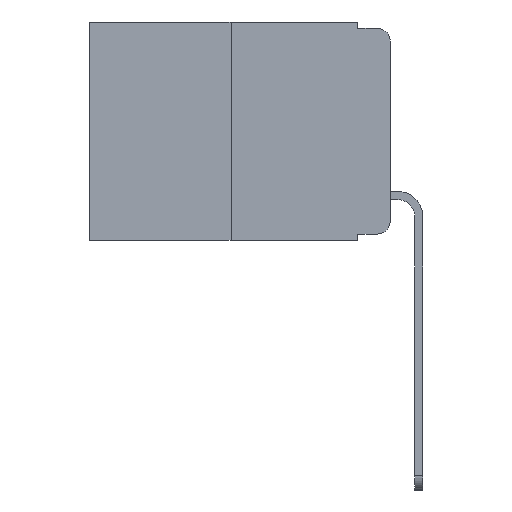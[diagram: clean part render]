
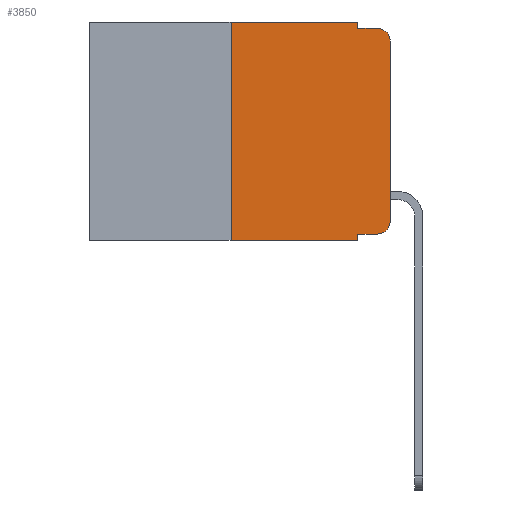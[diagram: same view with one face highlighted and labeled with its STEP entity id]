
A CAD part, left-side view. The second image highlights one B-rep face of the part: STEP entity #3850.
In plain terms, the highlighted planar face has unit normal (-1, 0, 0).
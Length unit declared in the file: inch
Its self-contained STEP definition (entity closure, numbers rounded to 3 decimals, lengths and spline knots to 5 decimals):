
#22 = VERTEX_POINT ( 'NONE', #5434 ) ;
#268 = LINE ( 'NONE', #22617, #21982 ) ;
#506 = CARTESIAN_POINT ( 'NONE',  ( 0., 0.051, -0.01 ) ) ;
#622 = EDGE_CURVE ( 'NONE', #5404, #12335, #5553, .T. ) ;
#743 = CARTESIAN_POINT ( 'NONE',  ( 0., 0.02, -0.333 ) ) ;
#933 = VERTEX_POINT ( 'NONE', #16867 ) ;
#1310 = LINE ( 'NONE', #3900, #15167 ) ;
#1451 = CARTESIAN_POINT ( 'NONE',  ( 0., 0.02, -0.313 ) ) ;
#2582 = CARTESIAN_POINT ( 'NONE',  ( 0., 0.051, -0.333 ) ) ;
#2832 = EDGE_CURVE ( 'NONE', #20714, #9793, #21020, .T. ) ;
#3211 = DIRECTION ( 'NONE',  ( 0., 0., -1. ) ) ;
#3547 = VERTEX_POINT ( 'NONE', #15795 ) ;
#3850 = ADVANCED_FACE ( 'NONE', ( #6837 ), #14515, .F. ) ;
#3899 = LINE ( 'NONE', #9962, #21106 ) ;
#3900 = CARTESIAN_POINT ( 'NONE',  ( 0., 0., 0. ) ) ;
#3973 = CARTESIAN_POINT ( 'NONE',  ( 0., 0., -0.313 ) ) ;
#4809 = CARTESIAN_POINT ( 'NONE',  ( 0., 0.02, -0.03 ) ) ;
#4933 = VECTOR ( 'NONE', #21950, 39.37008 ) ;
#5178 = DIRECTION ( 'NONE',  ( 0., -1., 0. ) ) ;
#5259 = LINE ( 'NONE', #506, #13717 ) ;
#5337 = VERTEX_POINT ( 'NONE', #8022 ) ;
#5404 = VERTEX_POINT ( 'NONE', #743 ) ;
#5434 = CARTESIAN_POINT ( 'NONE',  ( 0., 0.02, -0.01 ) ) ;
#5553 = CIRCLE ( 'NONE', #9701, 0.02 ) ;
#5694 = LINE ( 'NONE', #6574, #15062 ) ;
#6097 = CARTESIAN_POINT ( 'NONE',  ( 0., 0.051, -0.343 ) ) ;
#6574 = CARTESIAN_POINT ( 'NONE',  ( 0., 0.473, -0.343 ) ) ;
#6596 = DIRECTION ( 'NONE',  ( 0., 0., -1. ) ) ;
#6765 = DIRECTION ( 'NONE',  ( -1., 0., 0. ) ) ;
#6837 = FACE_OUTER_BOUND ( 'NONE', #8541, .T. ) ;
#7062 = ORIENTED_EDGE ( 'NONE', *, *, #21524, .F. ) ;
#7577 = DIRECTION ( 'NONE',  ( 0., 0., 1. ) ) ;
#7895 = EDGE_CURVE ( 'NONE', #20714, #5404, #268, .T. ) ;
#8022 = CARTESIAN_POINT ( 'NONE',  ( 0., 0.25, -0.343 ) ) ;
#8454 = CARTESIAN_POINT ( 'NONE',  ( 0., 0.051, -0.01 ) ) ;
#8541 = EDGE_LOOP ( 'NONE', ( #9739, #22229, #9077, #12948, #7062, #13990, #13149, #9765, #13218, #19068 ) ) ;
#8780 = DIRECTION ( 'NONE',  ( -1., 0., 0. ) ) ;
#9077 = ORIENTED_EDGE ( 'NONE', *, *, #10217, .F. ) ;
#9701 = AXIS2_PLACEMENT_3D ( 'NONE', #1451, #8780, #3211 ) ;
#9739 = ORIENTED_EDGE ( 'NONE', *, *, #19804, .T. ) ;
#9765 = ORIENTED_EDGE ( 'NONE', *, *, #2832, .F. ) ;
#9793 = VERTEX_POINT ( 'NONE', #6097 ) ;
#9962 = CARTESIAN_POINT ( 'NONE',  ( 0., 0.051, 0. ) ) ;
#10217 = EDGE_CURVE ( 'NONE', #16888, #22, #5259, .T. ) ;
#10586 = CARTESIAN_POINT ( 'NONE',  ( 0., 0.25, 0. ) ) ;
#10995 = DIRECTION ( 'NONE',  ( 1., 0., 0. ) ) ;
#11009 = CIRCLE ( 'NONE', #17565, 0.02 ) ;
#11788 = DIRECTION ( 'NONE',  ( 0., -1., 0. ) ) ;
#11918 = EDGE_CURVE ( 'NONE', #3547, #16888, #3899, .T. ) ;
#12335 = VERTEX_POINT ( 'NONE', #3973 ) ;
#12870 = EDGE_CURVE ( 'NONE', #5337, #22845, #16311, .T. ) ;
#12948 = ORIENTED_EDGE ( 'NONE', *, *, #11918, .F. ) ;
#13149 = ORIENTED_EDGE ( 'NONE', *, *, #22579, .T. ) ;
#13218 = ORIENTED_EDGE ( 'NONE', *, *, #7895, .T. ) ;
#13683 = DIRECTION ( 'NONE',  ( 0., -1., 0. ) ) ;
#13717 = VECTOR ( 'NONE', #18542, 39.37008 ) ;
#13990 = ORIENTED_EDGE ( 'NONE', *, *, #12870, .F. ) ;
#14515 = PLANE ( 'NONE',  #19475 ) ;
#14674 = DIRECTION ( 'NONE',  ( 0., 0., -1. ) ) ;
#14874 = VECTOR ( 'NONE', #19706, 39.37008 ) ;
#15062 = VECTOR ( 'NONE', #11788, 39.37008 ) ;
#15167 = VECTOR ( 'NONE', #7577, 39.37008 ) ;
#15721 = EDGE_CURVE ( 'NONE', #933, #22, #11009, .T. ) ;
#15795 = CARTESIAN_POINT ( 'NONE',  ( 0., 0.051, 0. ) ) ;
#15952 = VECTOR ( 'NONE', #5178, 39.37008 ) ;
#16178 = CARTESIAN_POINT ( 'NONE',  ( 0., 0.25, 0. ) ) ;
#16311 = LINE ( 'NONE', #10586, #14874 ) ;
#16867 = CARTESIAN_POINT ( 'NONE',  ( 0., 0., -0.03 ) ) ;
#16888 = VERTEX_POINT ( 'NONE', #8454 ) ;
#17565 = AXIS2_PLACEMENT_3D ( 'NONE', #4809, #6765, #21222 ) ;
#18149 = CARTESIAN_POINT ( 'NONE',  ( 0., 0.473, 0. ) ) ;
#18542 = DIRECTION ( 'NONE',  ( 0., -1., 0. ) ) ;
#19068 = ORIENTED_EDGE ( 'NONE', *, *, #622, .T. ) ;
#19475 = AXIS2_PLACEMENT_3D ( 'NONE', #18149, #10995, #14674 ) ;
#19706 = DIRECTION ( 'NONE',  ( 0., 0., 1. ) ) ;
#19804 = EDGE_CURVE ( 'NONE', #12335, #933, #1310, .T. ) ;
#20690 = LINE ( 'NONE', #23264, #15952 ) ;
#20714 = VERTEX_POINT ( 'NONE', #2582 ) ;
#21020 = LINE ( 'NONE', #22235, #4933 ) ;
#21106 = VECTOR ( 'NONE', #6596, 39.37008 ) ;
#21222 = DIRECTION ( 'NONE',  ( 0., 0., -1. ) ) ;
#21524 = EDGE_CURVE ( 'NONE', #22845, #3547, #20690, .T. ) ;
#21950 = DIRECTION ( 'NONE',  ( 0., 0., -1. ) ) ;
#21982 = VECTOR ( 'NONE', #13683, 39.37008 ) ;
#22229 = ORIENTED_EDGE ( 'NONE', *, *, #15721, .T. ) ;
#22235 = CARTESIAN_POINT ( 'NONE',  ( 0., 0.051, 0. ) ) ;
#22579 = EDGE_CURVE ( 'NONE', #5337, #9793, #5694, .T. ) ;
#22617 = CARTESIAN_POINT ( 'NONE',  ( 0., 0.051, -0.333 ) ) ;
#22845 = VERTEX_POINT ( 'NONE', #16178 ) ;
#23264 = CARTESIAN_POINT ( 'NONE',  ( 0., 0.473, 0. ) ) ;
